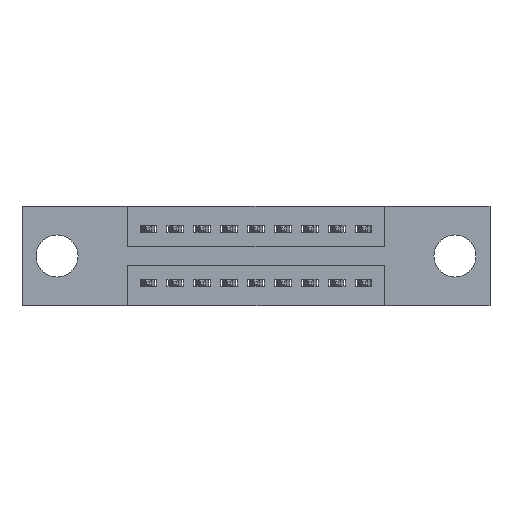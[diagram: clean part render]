
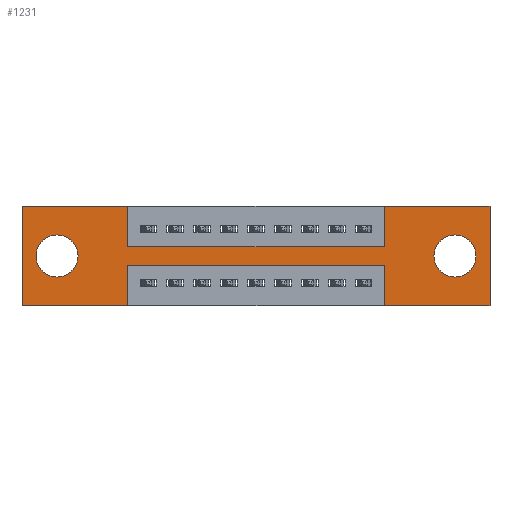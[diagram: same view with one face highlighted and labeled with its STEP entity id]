
A CAD part, front view. The second image highlights one B-rep face of the part: STEP entity #1231.
In plain terms, the highlighted planar face has unit normal (0, -1, 0).
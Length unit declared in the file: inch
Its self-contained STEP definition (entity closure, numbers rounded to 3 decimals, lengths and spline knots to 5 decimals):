
#129 = LINE ( 'NONE', #1158, #6225 ) ;
#404 = CARTESIAN_POINT ( 'NONE',  ( 0.13, 0., -0.185 ) ) ;
#481 = FACE_BOUND ( 'NONE', #7323, .T. ) ;
#594 = CARTESIAN_POINT ( 'NONE',  ( 1.3425, 0., -0.22 ) ) ;
#854 = CARTESIAN_POINT ( 'NONE',  ( 1.605, 0., -0.263 ) ) ;
#1019 = CARTESIAN_POINT ( 'NONE',  ( 1.3425, 0., -0.37 ) ) ;
#1082 = EDGE_CURVE ( 'NONE', #5155, #10065, #2970, .T. ) ;
#1125 = DIRECTION ( 'NONE',  ( 1., 0., 0. ) ) ;
#1158 = CARTESIAN_POINT ( 'NONE',  ( 0., 0., -0.37 ) ) ;
#1173 = CARTESIAN_POINT ( 'NONE',  ( 0.3925, 0., -0.22 ) ) ;
#1231 = ADVANCED_FACE ( 'NONE', ( #2239, #481, #4126 ), #4178, .T. ) ;
#1320 = LINE ( 'NONE', #2167, #10538 ) ;
#1354 = VERTEX_POINT ( 'NONE', #3317 ) ;
#1375 = EDGE_CURVE ( 'NONE', #4305, #2562, #8884, .T. ) ;
#1398 = DIRECTION ( 'NONE',  ( 0., 0., 1. ) ) ;
#1520 = LINE ( 'NONE', #9681, #11174 ) ;
#1605 = EDGE_CURVE ( 'NONE', #11679, #1354, #1320, .T. ) ;
#1612 = VERTEX_POINT ( 'NONE', #3248 ) ;
#1652 = CARTESIAN_POINT ( 'NONE',  ( 0.3925, 0., 0. ) ) ;
#1657 = ORIENTED_EDGE ( 'NONE', *, *, #7341, .T. ) ;
#1752 = DIRECTION ( 'NONE',  ( 0., 0., 1. ) ) ;
#1835 = CARTESIAN_POINT ( 'NONE',  ( 0.3925, 0., 0. ) ) ;
#1855 = EDGE_LOOP ( 'NONE', ( #2317, #9883 ) ) ;
#1954 = VECTOR ( 'NONE', #11244, 39.37008 ) ;
#2167 = CARTESIAN_POINT ( 'NONE',  ( 1.3425, 0., 0. ) ) ;
#2224 = CARTESIAN_POINT ( 'NONE',  ( 1.605, 0., -0.185 ) ) ;
#2239 = FACE_BOUND ( 'NONE', #1855, .T. ) ;
#2317 = ORIENTED_EDGE ( 'NONE', *, *, #4842, .T. ) ;
#2458 = AXIS2_PLACEMENT_3D ( 'NONE', #5947, #9610, #11482 ) ;
#2473 = CIRCLE ( 'NONE', #3053, 0.078 ) ;
#2499 = ORIENTED_EDGE ( 'NONE', *, *, #10380, .F. ) ;
#2562 = VERTEX_POINT ( 'NONE', #11788 ) ;
#2594 = VERTEX_POINT ( 'NONE', #9003 ) ;
#2597 = VERTEX_POINT ( 'NONE', #854 ) ;
#2736 = DIRECTION ( 'NONE',  ( -1., 0., 0. ) ) ;
#2970 = LINE ( 'NONE', #11015, #10556 ) ;
#2983 = DIRECTION ( 'NONE',  ( -1., 0., 0. ) ) ;
#2986 = ORIENTED_EDGE ( 'NONE', *, *, #1605, .F. ) ;
#3053 = AXIS2_PLACEMENT_3D ( 'NONE', #10433, #11286, #4851 ) ;
#3212 = ORIENTED_EDGE ( 'NONE', *, *, #7298, .F. ) ;
#3248 = CARTESIAN_POINT ( 'NONE',  ( 0.13, 0., -0.107 ) ) ;
#3317 = CARTESIAN_POINT ( 'NONE',  ( 1.3425, 0., 0. ) ) ;
#3353 = DIRECTION ( 'NONE',  ( 0., 1., 0. ) ) ;
#3412 = CARTESIAN_POINT ( 'NONE',  ( 1.735, 0., -0.37 ) ) ;
#3459 = CARTESIAN_POINT ( 'NONE',  ( 0.3925, 0., -0.22 ) ) ;
#3741 = ORIENTED_EDGE ( 'NONE', *, *, #11032, .F. ) ;
#3864 = EDGE_CURVE ( 'NONE', #10508, #7138, #11682, .T. ) ;
#4010 = DIRECTION ( 'NONE',  ( 1., 0., 0. ) ) ;
#4017 = ORIENTED_EDGE ( 'NONE', *, *, #5048, .T. ) ;
#4088 = CARTESIAN_POINT ( 'NONE',  ( 0.3925, 0., -0.37 ) ) ;
#4126 = FACE_OUTER_BOUND ( 'NONE', #8122, .T. ) ;
#4156 = CARTESIAN_POINT ( 'NONE',  ( 0., 0., 0. ) ) ;
#4178 = PLANE ( 'NONE',  #2458 ) ;
#4305 = VERTEX_POINT ( 'NONE', #9539 ) ;
#4351 = EDGE_CURVE ( 'NONE', #2597, #8973, #9608, .T. ) ;
#4386 = CARTESIAN_POINT ( 'NONE',  ( 0.3925, 0., -0.37 ) ) ;
#4832 = AXIS2_PLACEMENT_3D ( 'NONE', #5952, #5892, #1398 ) ;
#4833 = AXIS2_PLACEMENT_3D ( 'NONE', #404, #3353, #10553 ) ;
#4842 = EDGE_CURVE ( 'NONE', #8973, #2597, #2473, .T. ) ;
#4848 = VECTOR ( 'NONE', #7619, 39.37008 ) ;
#4851 = DIRECTION ( 'NONE',  ( 0., 0., -1. ) ) ;
#4930 = CARTESIAN_POINT ( 'NONE',  ( 1.3425, 0., -0.37 ) ) ;
#5048 = EDGE_CURVE ( 'NONE', #1612, #2594, #5598, .T. ) ;
#5060 = VERTEX_POINT ( 'NONE', #7783 ) ;
#5116 = ORIENTED_EDGE ( 'NONE', *, *, #3864, .F. ) ;
#5138 = EDGE_CURVE ( 'NONE', #2562, #10508, #9833, .T. ) ;
#5155 = VERTEX_POINT ( 'NONE', #3412 ) ;
#5332 = ORIENTED_EDGE ( 'NONE', *, *, #1082, .F. ) ;
#5594 = CARTESIAN_POINT ( 'NONE',  ( 1.735, 0., 0. ) ) ;
#5598 = CIRCLE ( 'NONE', #4833, 0.078 ) ;
#5713 = DIRECTION ( 'NONE',  ( -1., 0., 0. ) ) ;
#5737 = LINE ( 'NONE', #9399, #7377 ) ;
#5892 = DIRECTION ( 'NONE',  ( 0., 1., 0. ) ) ;
#5947 = CARTESIAN_POINT ( 'NONE',  ( 0., 0., -0.37 ) ) ;
#5952 = CARTESIAN_POINT ( 'NONE',  ( 0.13, 0., -0.185 ) ) ;
#6017 = ORIENTED_EDGE ( 'NONE', *, *, #1375, .F. ) ;
#6139 = LINE ( 'NONE', #4386, #6605 ) ;
#6225 = VECTOR ( 'NONE', #5713, 39.37008 ) ;
#6254 = CARTESIAN_POINT ( 'NONE',  ( 1.605, 0., -0.107 ) ) ;
#6285 = CARTESIAN_POINT ( 'NONE',  ( 0., 0., 0. ) ) ;
#6605 = VECTOR ( 'NONE', #9825, 39.37008 ) ;
#6711 = VECTOR ( 'NONE', #1752, 39.37008 ) ;
#6766 = DIRECTION ( 'NONE',  ( 0., 0., 1. ) ) ;
#6830 = VERTEX_POINT ( 'NONE', #4088 ) ;
#6987 = DIRECTION ( 'NONE',  ( 1., 0., 0. ) ) ;
#7041 = ORIENTED_EDGE ( 'NONE', *, *, #10129, .F. ) ;
#7138 = VERTEX_POINT ( 'NONE', #10346 ) ;
#7298 = EDGE_CURVE ( 'NONE', #7138, #11679, #1520, .T. ) ;
#7323 = EDGE_LOOP ( 'NONE', ( #4017, #1657 ) ) ;
#7341 = EDGE_CURVE ( 'NONE', #2594, #1612, #11561, .T. ) ;
#7377 = VECTOR ( 'NONE', #1125, 39.37008 ) ;
#7498 = AXIS2_PLACEMENT_3D ( 'NONE', #2224, #11421, #8695 ) ;
#7569 = EDGE_CURVE ( 'NONE', #5060, #5155, #8458, .T. ) ;
#7580 = LINE ( 'NONE', #1173, #10868 ) ;
#7619 = DIRECTION ( 'NONE',  ( 0., 0., -1. ) ) ;
#7693 = VECTOR ( 'NONE', #6987, 39.37008 ) ;
#7778 = ORIENTED_EDGE ( 'NONE', *, *, #7569, .F. ) ;
#7783 = CARTESIAN_POINT ( 'NONE',  ( 1.735, 0., 0. ) ) ;
#7955 = VERTEX_POINT ( 'NONE', #594 ) ;
#8084 = ORIENTED_EDGE ( 'NONE', *, *, #9776, .F. ) ;
#8122 = EDGE_LOOP ( 'NONE', ( #2499, #10431, #8084, #5332, #7778, #7041, #2986, #3212, #5116, #8845, #6017, #3741 ) ) ;
#8406 = LINE ( 'NONE', #4930, #1954 ) ;
#8438 = VECTOR ( 'NONE', #9754, 39.37008 ) ;
#8458 = LINE ( 'NONE', #5594, #4848 ) ;
#8695 = DIRECTION ( 'NONE',  ( 0., 0., -1. ) ) ;
#8845 = ORIENTED_EDGE ( 'NONE', *, *, #5138, .F. ) ;
#8884 = LINE ( 'NONE', #6285, #6711 ) ;
#8973 = VERTEX_POINT ( 'NONE', #6254 ) ;
#8986 = VERTEX_POINT ( 'NONE', #3459 ) ;
#9003 = CARTESIAN_POINT ( 'NONE',  ( 0.13, 0., -0.263 ) ) ;
#9399 = CARTESIAN_POINT ( 'NONE',  ( 0., 0., 0. ) ) ;
#9539 = CARTESIAN_POINT ( 'NONE',  ( 0., 0., -0.37 ) ) ;
#9608 = CIRCLE ( 'NONE', #7498, 0.078 ) ;
#9610 = DIRECTION ( 'NONE',  ( 0., -1., 0. ) ) ;
#9657 = CARTESIAN_POINT ( 'NONE',  ( 1.3425, 0., -0.15 ) ) ;
#9681 = CARTESIAN_POINT ( 'NONE',  ( 0.3925, 0., -0.15 ) ) ;
#9754 = DIRECTION ( 'NONE',  ( 0., 0., -1. ) ) ;
#9776 = EDGE_CURVE ( 'NONE', #10065, #7955, #8406, .T. ) ;
#9825 = DIRECTION ( 'NONE',  ( 0., 0., -1. ) ) ;
#9833 = LINE ( 'NONE', #4156, #7693 ) ;
#9883 = ORIENTED_EDGE ( 'NONE', *, *, #4351, .T. ) ;
#10065 = VERTEX_POINT ( 'NONE', #1019 ) ;
#10129 = EDGE_CURVE ( 'NONE', #1354, #5060, #5737, .T. ) ;
#10346 = CARTESIAN_POINT ( 'NONE',  ( 0.3925, 0., -0.15 ) ) ;
#10380 = EDGE_CURVE ( 'NONE', #8986, #6830, #6139, .T. ) ;
#10431 = ORIENTED_EDGE ( 'NONE', *, *, #11944, .F. ) ;
#10433 = CARTESIAN_POINT ( 'NONE',  ( 1.605, 0., -0.185 ) ) ;
#10508 = VERTEX_POINT ( 'NONE', #1835 ) ;
#10538 = VECTOR ( 'NONE', #6766, 39.37008 ) ;
#10553 = DIRECTION ( 'NONE',  ( 0., 0., 1. ) ) ;
#10556 = VECTOR ( 'NONE', #2736, 39.37008 ) ;
#10868 = VECTOR ( 'NONE', #2983, 39.37008 ) ;
#11015 = CARTESIAN_POINT ( 'NONE',  ( 0., 0., -0.37 ) ) ;
#11032 = EDGE_CURVE ( 'NONE', #6830, #4305, #129, .T. ) ;
#11174 = VECTOR ( 'NONE', #4010, 39.37008 ) ;
#11244 = DIRECTION ( 'NONE',  ( 0., 0., 1. ) ) ;
#11286 = DIRECTION ( 'NONE',  ( 0., 1., 0. ) ) ;
#11421 = DIRECTION ( 'NONE',  ( 0., 1., 0. ) ) ;
#11482 = DIRECTION ( 'NONE',  ( 0., 0., -1. ) ) ;
#11561 = CIRCLE ( 'NONE', #4832, 0.078 ) ;
#11679 = VERTEX_POINT ( 'NONE', #9657 ) ;
#11682 = LINE ( 'NONE', #1652, #8438 ) ;
#11788 = CARTESIAN_POINT ( 'NONE',  ( 0., 0., 0. ) ) ;
#11944 = EDGE_CURVE ( 'NONE', #7955, #8986, #7580, .T. ) ;
